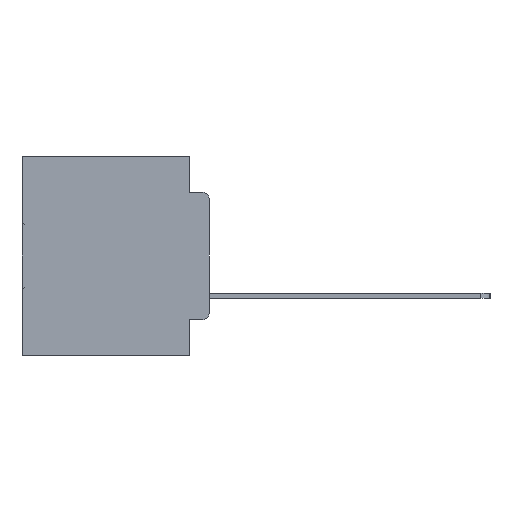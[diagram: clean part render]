
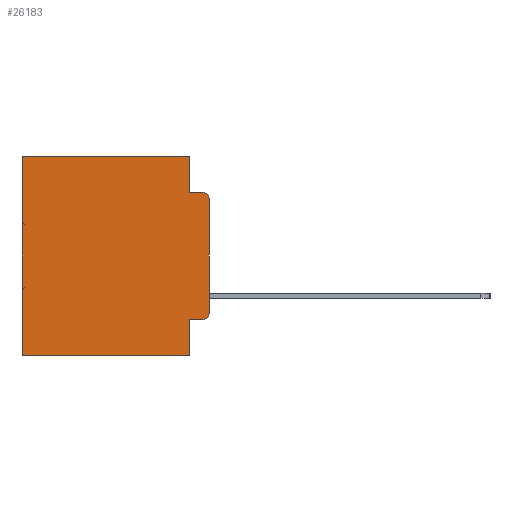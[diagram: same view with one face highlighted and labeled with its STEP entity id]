
A CAD part, left-side view. The second image highlights one B-rep face of the part: STEP entity #26183.
In plain terms, the highlighted planar face has unit normal (-1, 0, 0).
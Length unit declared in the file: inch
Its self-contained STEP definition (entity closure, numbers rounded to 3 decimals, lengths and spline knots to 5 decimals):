
#284 = CARTESIAN_POINT ( 'NONE',  ( 0.298, 0.051, -0.5 ) ) ;
#516 = VECTOR ( 'NONE', #26667, 39.37008 ) ;
#578 = DIRECTION ( 'NONE',  ( 1., 0., 0. ) ) ;
#610 = CARTESIAN_POINT ( 'NONE',  ( 0.298, 0.02, -0.0885 ) ) ;
#743 = AXIS2_PLACEMENT_3D ( 'NONE', #10513, #28994, #13166 ) ;
#1009 = EDGE_CURVE ( 'NONE', #28828, #21418, #11760, .T. ) ;
#1278 = CIRCLE ( 'NONE', #743, 0.02 ) ;
#3640 = CARTESIAN_POINT ( 'NONE',  ( 0.298, 0.051, -0.0885 ) ) ;
#4060 = LINE ( 'NONE', #18326, #31296 ) ;
#4512 = VECTOR ( 'NONE', #7688, 39.37008 ) ;
#4724 = VECTOR ( 'NONE', #31201, 39.37008 ) ;
#5349 = ORIENTED_EDGE ( 'NONE', *, *, #28677, .F. ) ;
#5661 = VECTOR ( 'NONE', #30517, 39.37008 ) ;
#5849 = EDGE_CURVE ( 'NONE', #24449, #10882, #6162, .T. ) ;
#6101 = DIRECTION ( 'NONE',  ( 0., 0., -1. ) ) ;
#6162 = LINE ( 'NONE', #26222, #4512 ) ;
#6465 = EDGE_CURVE ( 'NONE', #18276, #30319, #4060, .T. ) ;
#6868 = EDGE_CURVE ( 'NONE', #8859, #30680, #20593, .T. ) ;
#7020 = EDGE_CURVE ( 'NONE', #10882, #30319, #1278, .T. ) ;
#7354 = VECTOR ( 'NONE', #19118, 39.37008 ) ;
#7379 = CARTESIAN_POINT ( 'NONE',  ( 0.298, 0.051, 0. ) ) ;
#7688 = DIRECTION ( 'NONE',  ( 0., -1., 0. ) ) ;
#7971 = CARTESIAN_POINT ( 'NONE',  ( 0.298, 0.473, 0. ) ) ;
#8076 = DIRECTION ( 'NONE',  ( -1., 0., 0. ) ) ;
#8859 = VERTEX_POINT ( 'NONE', #3640 ) ;
#9014 = LINE ( 'NONE', #32208, #7354 ) ;
#9180 = CARTESIAN_POINT ( 'NONE',  ( 0.298, 0.473, -0.5 ) ) ;
#10078 = ORIENTED_EDGE ( 'NONE', *, *, #22279, .T. ) ;
#10513 = CARTESIAN_POINT ( 'NONE',  ( 0.298, 0.02, -0.3915 ) ) ;
#10525 = VECTOR ( 'NONE', #6101, 39.37008 ) ;
#10646 = FACE_OUTER_BOUND ( 'NONE', #23718, .T. ) ;
#10882 = VERTEX_POINT ( 'NONE', #20064 ) ;
#11107 = CARTESIAN_POINT ( 'NONE',  ( 0.298, 0., 0. ) ) ;
#11760 = LINE ( 'NONE', #33719, #4724 ) ;
#12710 = CIRCLE ( 'NONE', #33792, 0.02 ) ;
#13116 = ORIENTED_EDGE ( 'NONE', *, *, #5849, .T. ) ;
#13166 = DIRECTION ( 'NONE',  ( 0., 0., -1. ) ) ;
#14577 = EDGE_CURVE ( 'NONE', #18276, #30680, #12710, .T. ) ;
#14606 = LINE ( 'NONE', #18232, #516 ) ;
#16442 = PLANE ( 'NONE',  #28145 ) ;
#16843 = ORIENTED_EDGE ( 'NONE', *, *, #17637, .F. ) ;
#17637 = EDGE_CURVE ( 'NONE', #28828, #8859, #23383, .T. ) ;
#18125 = CARTESIAN_POINT ( 'NONE',  ( 0.298, 0., -0.1085 ) ) ;
#18232 = CARTESIAN_POINT ( 'NONE',  ( 0.298, 0.051, 0. ) ) ;
#18276 = VERTEX_POINT ( 'NONE', #18125 ) ;
#18326 = CARTESIAN_POINT ( 'NONE',  ( 0.298, 0., 0. ) ) ;
#19118 = DIRECTION ( 'NONE',  ( 0., 1., 0. ) ) ;
#19138 = DIRECTION ( 'NONE',  ( 0., 0., -1. ) ) ;
#20064 = CARTESIAN_POINT ( 'NONE',  ( 0.298, 0.02, -0.4115 ) ) ;
#20127 = ORIENTED_EDGE ( 'NONE', *, *, #6868, .F. ) ;
#20593 = LINE ( 'NONE', #27892, #5661 ) ;
#20755 = ORIENTED_EDGE ( 'NONE', *, *, #7020, .T. ) ;
#20932 = ORIENTED_EDGE ( 'NONE', *, *, #33065, .F. ) ;
#21418 = VERTEX_POINT ( 'NONE', #7971 ) ;
#22138 = ORIENTED_EDGE ( 'NONE', *, *, #14577, .T. ) ;
#22279 = EDGE_CURVE ( 'NONE', #21418, #32104, #23831, .T. ) ;
#23383 = LINE ( 'NONE', #7379, #29508 ) ;
#23718 = EDGE_LOOP ( 'NONE', ( #23747, #22138, #20127, #16843, #27403, #10078, #20932, #5349, #13116, #20755 ) ) ;
#23747 = ORIENTED_EDGE ( 'NONE', *, *, #6465, .F. ) ;
#23831 = LINE ( 'NONE', #24644, #10525 ) ;
#23998 = CARTESIAN_POINT ( 'NONE',  ( 0.298, 0.02, -0.1085 ) ) ;
#24449 = VERTEX_POINT ( 'NONE', #28267 ) ;
#24644 = CARTESIAN_POINT ( 'NONE',  ( 0.298, 0.473, 0. ) ) ;
#25932 = DIRECTION ( 'NONE',  ( 0., 0., -1. ) ) ;
#26183 = ADVANCED_FACE ( 'NONE', ( #10646 ), #16442, .F. ) ;
#26222 = CARTESIAN_POINT ( 'NONE',  ( 0.298, 0.051, -0.4115 ) ) ;
#26609 = DIRECTION ( 'NONE',  ( 0., 0., -1. ) ) ;
#26667 = DIRECTION ( 'NONE',  ( 0., 0., -1. ) ) ;
#27403 = ORIENTED_EDGE ( 'NONE', *, *, #1009, .T. ) ;
#27892 = CARTESIAN_POINT ( 'NONE',  ( 0.298, 0.051, -0.0885 ) ) ;
#28064 = CARTESIAN_POINT ( 'NONE',  ( 0.298, 0., -0.3915 ) ) ;
#28145 = AXIS2_PLACEMENT_3D ( 'NONE', #11107, #578, #19138 ) ;
#28267 = CARTESIAN_POINT ( 'NONE',  ( 0.298, 0.051, -0.4115 ) ) ;
#28677 = EDGE_CURVE ( 'NONE', #24449, #33624, #14606, .T. ) ;
#28828 = VERTEX_POINT ( 'NONE', #32495 ) ;
#28994 = DIRECTION ( 'NONE',  ( -1., 0., 0. ) ) ;
#29508 = VECTOR ( 'NONE', #25932, 39.37008 ) ;
#30319 = VERTEX_POINT ( 'NONE', #28064 ) ;
#30517 = DIRECTION ( 'NONE',  ( 0., -1., 0. ) ) ;
#30680 = VERTEX_POINT ( 'NONE', #610 ) ;
#31201 = DIRECTION ( 'NONE',  ( 0., 1., 0. ) ) ;
#31296 = VECTOR ( 'NONE', #31440, 39.37008 ) ;
#31440 = DIRECTION ( 'NONE',  ( 0., 0., -1. ) ) ;
#32104 = VERTEX_POINT ( 'NONE', #9180 ) ;
#32208 = CARTESIAN_POINT ( 'NONE',  ( 0.298, 0., -0.5 ) ) ;
#32495 = CARTESIAN_POINT ( 'NONE',  ( 0.298, 0.051, 0. ) ) ;
#33065 = EDGE_CURVE ( 'NONE', #33624, #32104, #9014, .T. ) ;
#33624 = VERTEX_POINT ( 'NONE', #284 ) ;
#33719 = CARTESIAN_POINT ( 'NONE',  ( 0.298, 0., 0. ) ) ;
#33792 = AXIS2_PLACEMENT_3D ( 'NONE', #23998, #8076, #26609 ) ;
